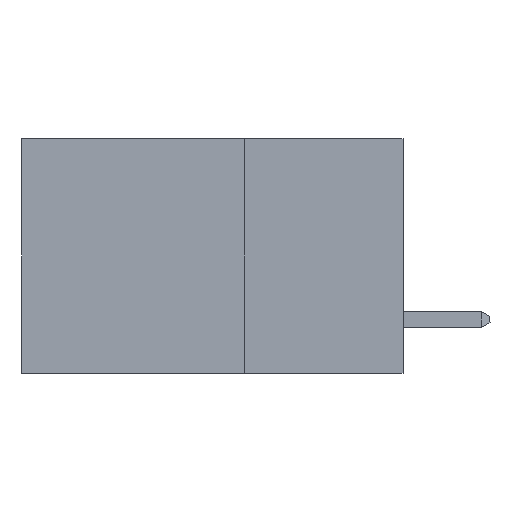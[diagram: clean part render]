
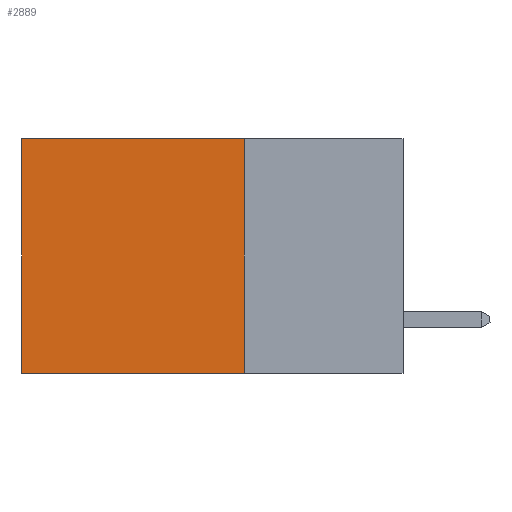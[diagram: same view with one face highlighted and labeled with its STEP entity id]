
A CAD part, left-side view. The second image highlights one B-rep face of the part: STEP entity #2889.
In plain terms, the highlighted planar face has unit normal (-1, 0, 0).
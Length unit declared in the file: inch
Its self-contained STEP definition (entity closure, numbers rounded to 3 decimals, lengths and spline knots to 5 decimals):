
#710 = DIRECTION ( 'NONE',  ( 0., 0., -1. ) ) ;
#956 = ORIENTED_EDGE ( 'NONE', *, *, #22484, .F. ) ;
#2889 = ADVANCED_FACE ( 'NONE', ( #23774 ), #23066, .F. ) ;
#3866 = CARTESIAN_POINT ( 'NONE',  ( 0.2875, 0.6, -0.37 ) ) ;
#3980 = VECTOR ( 'NONE', #18297, 39.37008 ) ;
#4494 = DIRECTION ( 'NONE',  ( 1., 0., 0. ) ) ;
#5357 = EDGE_CURVE ( 'NONE', #21308, #6621, #18488, .T. ) ;
#6621 = VERTEX_POINT ( 'NONE', #3866 ) ;
#7429 = DIRECTION ( 'NONE',  ( 0., 0., -1. ) ) ;
#7725 = DIRECTION ( 'NONE',  ( 0., 1., 0. ) ) ;
#8578 = VECTOR ( 'NONE', #7725, 39.37008 ) ;
#9430 = VECTOR ( 'NONE', #16245, 39.37008 ) ;
#10381 = AXIS2_PLACEMENT_3D ( 'NONE', #21253, #4494, #710 ) ;
#12651 = CARTESIAN_POINT ( 'NONE',  ( 0.2875, 0.25, 0. ) ) ;
#14345 = CARTESIAN_POINT ( 'NONE',  ( 0.2875, 0.6, 0. ) ) ;
#14555 = ORIENTED_EDGE ( 'NONE', *, *, #19355, .T. ) ;
#14965 = EDGE_CURVE ( 'NONE', #15154, #6621, #22085, .T. ) ;
#15000 = EDGE_LOOP ( 'NONE', ( #20071, #21056, #956, #14555 ) ) ;
#15154 = VERTEX_POINT ( 'NONE', #22317 ) ;
#15271 = CARTESIAN_POINT ( 'NONE',  ( 0.2875, 0.25, 0. ) ) ;
#16245 = DIRECTION ( 'NONE',  ( 0., 0., -1. ) ) ;
#16976 = CARTESIAN_POINT ( 'NONE',  ( 0.2875, 0.25, -0.37 ) ) ;
#17667 = VECTOR ( 'NONE', #7429, 39.37008 ) ;
#18297 = DIRECTION ( 'NONE',  ( 0., 1., 0. ) ) ;
#18488 = LINE ( 'NONE', #16976, #8578 ) ;
#18857 = LINE ( 'NONE', #12651, #3980 ) ;
#18958 = CARTESIAN_POINT ( 'NONE',  ( 0.2875, 0.25, -0.37 ) ) ;
#19355 = EDGE_CURVE ( 'NONE', #23719, #15154, #18857, .T. ) ;
#20071 = ORIENTED_EDGE ( 'NONE', *, *, #14965, .T. ) ;
#20474 = CARTESIAN_POINT ( 'NONE',  ( 0.2875, 0.25, 0. ) ) ;
#21056 = ORIENTED_EDGE ( 'NONE', *, *, #5357, .F. ) ;
#21253 = CARTESIAN_POINT ( 'NONE',  ( 0.2875, 0.25, 0. ) ) ;
#21308 = VERTEX_POINT ( 'NONE', #18958 ) ;
#22085 = LINE ( 'NONE', #14345, #9430 ) ;
#22317 = CARTESIAN_POINT ( 'NONE',  ( 0.2875, 0.6, 0. ) ) ;
#22484 = EDGE_CURVE ( 'NONE', #23719, #21308, #22575, .T. ) ;
#22575 = LINE ( 'NONE', #20474, #17667 ) ;
#23066 = PLANE ( 'NONE',  #10381 ) ;
#23719 = VERTEX_POINT ( 'NONE', #15271 ) ;
#23774 = FACE_OUTER_BOUND ( 'NONE', #15000, .T. ) ;
